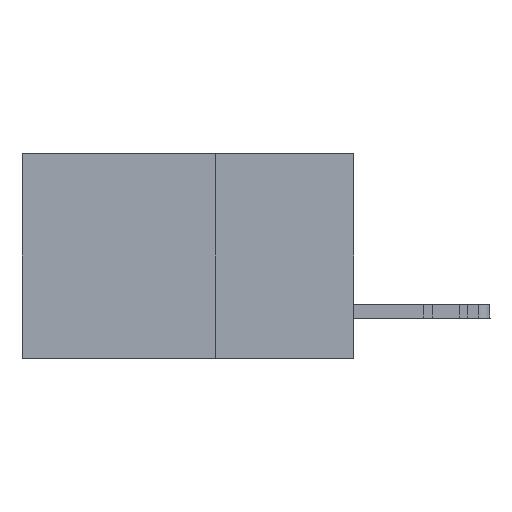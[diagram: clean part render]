
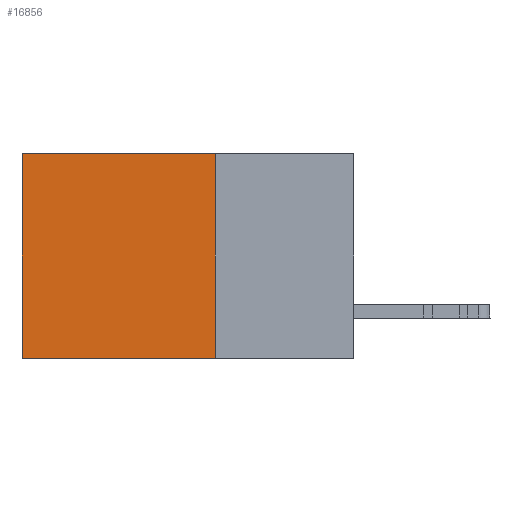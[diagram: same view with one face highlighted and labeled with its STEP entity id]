
A CAD part, left-side view. The second image highlights one B-rep face of the part: STEP entity #16856.
In plain terms, the highlighted planar face has unit normal (-1, 0, 0).
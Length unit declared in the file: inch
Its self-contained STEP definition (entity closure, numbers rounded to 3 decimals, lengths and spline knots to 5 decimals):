
#588 = EDGE_CURVE ( 'NONE', #15721, #15209, #23601, .T. ) ;
#1014 = CARTESIAN_POINT ( 'NONE',  ( 0.2875, 0.25, -0.37 ) ) ;
#1022 = FACE_OUTER_BOUND ( 'NONE', #2887, .T. ) ;
#2887 = EDGE_LOOP ( 'NONE', ( #36850, #6223, #14411, #28739 ) ) ;
#3608 = DIRECTION ( 'NONE',  ( 1., 0., 0. ) ) ;
#3818 = AXIS2_PLACEMENT_3D ( 'NONE', #10222, #3608, #19602 ) ;
#4051 = VECTOR ( 'NONE', #5047, 39.37008 ) ;
#4604 = DIRECTION ( 'NONE',  ( 0., 0., -1. ) ) ;
#5047 = DIRECTION ( 'NONE',  ( 0., 1., 0. ) ) ;
#5580 = LINE ( 'NONE', #9968, #30767 ) ;
#6223 = ORIENTED_EDGE ( 'NONE', *, *, #588, .F. ) ;
#6383 = LINE ( 'NONE', #22127, #10464 ) ;
#7915 = LINE ( 'NONE', #7989, #17146 ) ;
#7989 = CARTESIAN_POINT ( 'NONE',  ( 0.2875, 0.25, 0. ) ) ;
#8145 = DIRECTION ( 'NONE',  ( 0., 0., -1. ) ) ;
#9968 = CARTESIAN_POINT ( 'NONE',  ( 0.2875, 0.6, 0. ) ) ;
#10222 = CARTESIAN_POINT ( 'NONE',  ( 0.2875, 0.25, 0. ) ) ;
#10464 = VECTOR ( 'NONE', #35238, 39.37008 ) ;
#12237 = EDGE_CURVE ( 'NONE', #15551, #15209, #5580, .T. ) ;
#13361 = CARTESIAN_POINT ( 'NONE',  ( 0.2875, 0.25, -0.37 ) ) ;
#14411 = ORIENTED_EDGE ( 'NONE', *, *, #36205, .F. ) ;
#15209 = VERTEX_POINT ( 'NONE', #35572 ) ;
#15551 = VERTEX_POINT ( 'NONE', #39024 ) ;
#15721 = VERTEX_POINT ( 'NONE', #13361 ) ;
#16856 = ADVANCED_FACE ( 'NONE', ( #1022 ), #39311, .F. ) ;
#17146 = VECTOR ( 'NONE', #8145, 39.37008 ) ;
#19602 = DIRECTION ( 'NONE',  ( 0., 0., -1. ) ) ;
#22127 = CARTESIAN_POINT ( 'NONE',  ( 0.2875, 0.25, 0. ) ) ;
#23601 = LINE ( 'NONE', #1014, #4051 ) ;
#24847 = EDGE_CURVE ( 'NONE', #32112, #15551, #6383, .T. ) ;
#28739 = ORIENTED_EDGE ( 'NONE', *, *, #24847, .T. ) ;
#30767 = VECTOR ( 'NONE', #4604, 39.37008 ) ;
#32112 = VERTEX_POINT ( 'NONE', #35190 ) ;
#35190 = CARTESIAN_POINT ( 'NONE',  ( 0.2875, 0.25, 0. ) ) ;
#35238 = DIRECTION ( 'NONE',  ( 0., 1., 0. ) ) ;
#35572 = CARTESIAN_POINT ( 'NONE',  ( 0.2875, 0.6, -0.37 ) ) ;
#36205 = EDGE_CURVE ( 'NONE', #32112, #15721, #7915, .T. ) ;
#36850 = ORIENTED_EDGE ( 'NONE', *, *, #12237, .T. ) ;
#39024 = CARTESIAN_POINT ( 'NONE',  ( 0.2875, 0.6, 0. ) ) ;
#39311 = PLANE ( 'NONE',  #3818 ) ;
